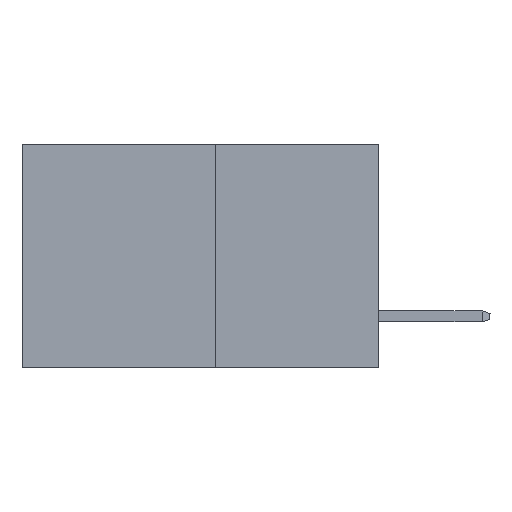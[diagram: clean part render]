
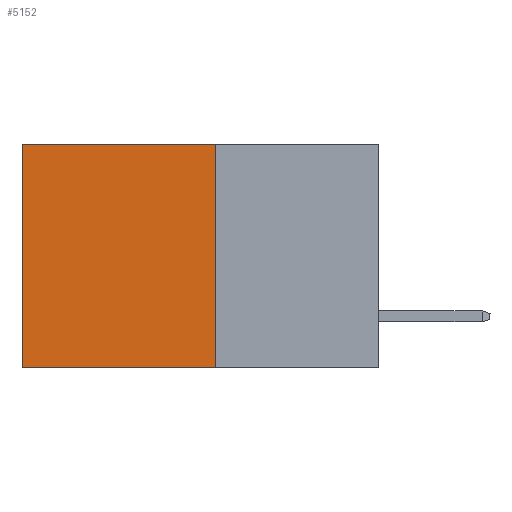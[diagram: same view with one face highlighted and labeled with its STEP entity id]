
A CAD part, left-side view. The second image highlights one B-rep face of the part: STEP entity #5152.
In plain terms, the highlighted planar face has unit normal (-1, 0, 0).
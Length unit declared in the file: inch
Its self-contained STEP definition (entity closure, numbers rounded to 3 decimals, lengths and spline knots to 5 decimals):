
#36 = DIRECTION ( 'NONE',  ( 0., 0., -1. ) ) ;
#77 = VERTEX_POINT ( 'NONE', #901 ) ;
#182 = CARTESIAN_POINT ( 'NONE',  ( 0.277, 0.59, -0.37 ) ) ;
#901 = CARTESIAN_POINT ( 'NONE',  ( 0.277, 0.59, -0.37 ) ) ;
#1001 = VERTEX_POINT ( 'NONE', #5057 ) ;
#1677 = VECTOR ( 'NONE', #2889, 39.37008 ) ;
#2141 = PLANE ( 'NONE',  #3738 ) ;
#2208 = EDGE_CURVE ( 'NONE', #4541, #1001, #6121, .T. ) ;
#2232 = CARTESIAN_POINT ( 'NONE',  ( 0.277, 0.27, -0.37 ) ) ;
#2367 = DIRECTION ( 'NONE',  ( 0., 1., 0. ) ) ;
#2404 = EDGE_CURVE ( 'NONE', #4541, #3472, #4085, .T. ) ;
#2804 = DIRECTION ( 'NONE',  ( 1., 0., 0. ) ) ;
#2886 = CARTESIAN_POINT ( 'NONE',  ( 0.277, 0.27, -0.37 ) ) ;
#2889 = DIRECTION ( 'NONE',  ( 0., 0., -1. ) ) ;
#3472 = VERTEX_POINT ( 'NONE', #6001 ) ;
#3666 = LINE ( 'NONE', #7354, #9145 ) ;
#3738 = AXIS2_PLACEMENT_3D ( 'NONE', #2232, #2804, #6952 ) ;
#3748 = EDGE_LOOP ( 'NONE', ( #6119, #6324, #8869, #8880 ) ) ;
#4085 = LINE ( 'NONE', #4802, #5781 ) ;
#4541 = VERTEX_POINT ( 'NONE', #8554 ) ;
#4802 = CARTESIAN_POINT ( 'NONE',  ( 0.277, 0.27, 0. ) ) ;
#4946 = FACE_OUTER_BOUND ( 'NONE', #3748, .T. ) ;
#5057 = CARTESIAN_POINT ( 'NONE',  ( 0.277, 0.27, -0.37 ) ) ;
#5152 = ADVANCED_FACE ( 'NONE', ( #4946 ), #2141, .F. ) ;
#5781 = VECTOR ( 'NONE', #7524, 39.37008 ) ;
#6001 = CARTESIAN_POINT ( 'NONE',  ( 0.277, 0.59, 0. ) ) ;
#6119 = ORIENTED_EDGE ( 'NONE', *, *, #8491, .T. ) ;
#6121 = LINE ( 'NONE', #2886, #1677 ) ;
#6301 = EDGE_CURVE ( 'NONE', #1001, #77, #3666, .T. ) ;
#6324 = ORIENTED_EDGE ( 'NONE', *, *, #6301, .F. ) ;
#6783 = VECTOR ( 'NONE', #36, 39.37008 ) ;
#6952 = DIRECTION ( 'NONE',  ( 0., 0., -1. ) ) ;
#7354 = CARTESIAN_POINT ( 'NONE',  ( 0.277, 0.27, -0.37 ) ) ;
#7524 = DIRECTION ( 'NONE',  ( 0., 1., 0. ) ) ;
#8460 = LINE ( 'NONE', #182, #6783 ) ;
#8491 = EDGE_CURVE ( 'NONE', #3472, #77, #8460, .T. ) ;
#8554 = CARTESIAN_POINT ( 'NONE',  ( 0.277, 0.27, 0. ) ) ;
#8869 = ORIENTED_EDGE ( 'NONE', *, *, #2208, .F. ) ;
#8880 = ORIENTED_EDGE ( 'NONE', *, *, #2404, .T. ) ;
#9145 = VECTOR ( 'NONE', #2367, 39.37008 ) ;
